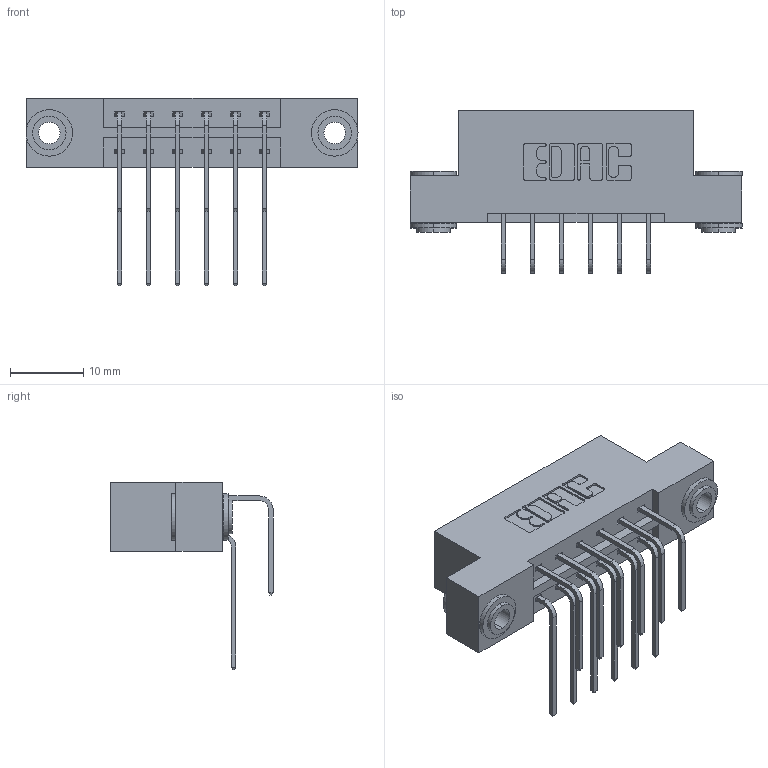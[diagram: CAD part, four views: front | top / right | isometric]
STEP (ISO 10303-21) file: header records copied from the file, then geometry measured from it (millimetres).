
FILE_DESCRIPTION (( 'STEP AP203' ), '1' );
FILE_NAME ('333-012-558-203.STEP', '2018-08-01T00:50:58', ( '' ), ( '' ), 'SwSTEP 2.0', 'SolidWorks 2016', '' );
FILE_SCHEMA (( 'CONFIG_CONTROL_DESIGN' ));
Length unit declared in the file: inch
Products named in the file (5): 345-292-001_558 559 Tail - 1; 345-292-001_558 Tail - 2; 345-250-002_345-250-002-102; 333-012-558-203; 333 Part_Flush - .156 Dia - TH
Assembly tree (15 placements, depth 2):
  333-012-558-203
    333 Part_Flush - .156 Dia - TH
    345-292-001_558 559 Tail - 1  x6
    345-292-001_558 Tail - 2  x6
    345-250-002_345-250-002-102  x2
Bounding box: 45.31 x 22.17 x 25.53 mm (x, y, z)
Volume: 4378.2 mm3; surface area: 5355 mm2
Topology: 15 solids, 15 shells, 800 faces, 2319 edges, 1526 vertices
Faces by surface type: plane 536, cylinder 256, cone 8
Entity records: 10950 total; most frequent: CARTESIAN_POINT 1884, ORIENTED_EDGE 1762, DIRECTION 1687, EDGE_CURVE 881, VECTOR 689, LINE 689, VERTEX_POINT 582, AXIS2_PLACEMENT_3D 499
